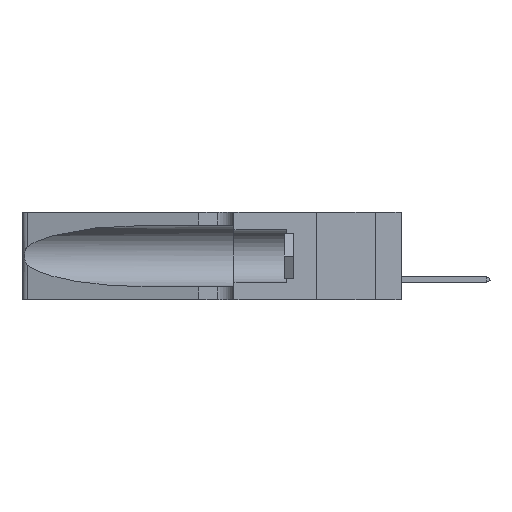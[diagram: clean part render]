
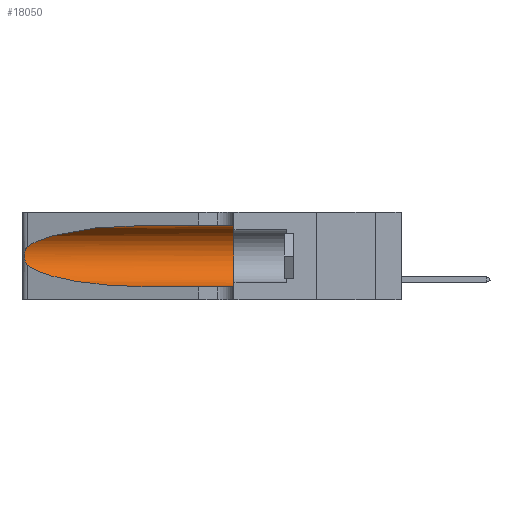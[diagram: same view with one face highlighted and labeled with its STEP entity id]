
A CAD part, left-side view. The second image highlights one B-rep face of the part: STEP entity #18050.
In plain terms, the highlighted cylindrical face has radius 3.308 mm (diameter 6.617 mm), a partial arc.
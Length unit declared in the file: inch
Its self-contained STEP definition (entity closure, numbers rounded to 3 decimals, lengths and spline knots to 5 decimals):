
#1642 = CIRCLE ( 'NONE', #11534, 0.13025 ) ;
#1746 = CARTESIAN_POINT ( 'NONE',  ( 0.26075, 1.23896, 0.19203 ) ) ;
#3138 = VERTEX_POINT ( 'NONE', #9955 ) ;
#3165 = EDGE_CURVE ( 'NONE', #3138, #22625, #1642, .T. ) ;
#3454 = VERTEX_POINT ( 'NONE', #5113 ) ;
#3626 = CARTESIAN_POINT ( 'NONE',  ( 0.25789, 1.23486, 0.15765 ) ) ;
#4269 = ORIENTED_EDGE ( 'NONE', *, *, #8485, .T. ) ;
#5087 = CARTESIAN_POINT ( 'NONE',  ( 0.25487, 1.22718, 0.22369 ) ) ;
#5113 = CARTESIAN_POINT ( 'NONE',  ( 0.25487, 1.22718, 0.22369 ) ) ;
#5138 = VERTEX_POINT ( 'NONE', #9258 ) ;
#5312 = CARTESIAN_POINT ( 'NONE',  ( 0.26018, 1.23835, 0.19895 ) ) ;
#5624 = CARTESIAN_POINT ( 'NONE',  ( 0.1305, 1.61858, 0.05475 ) ) ;
#5679 = ORIENTED_EDGE ( 'NONE', *, *, #8250, .F. ) ;
#5710 = DIRECTION ( 'NONE',  ( 0., -1., 0. ) ) ;
#6046 = LINE ( 'NONE', #5624, #17966 ) ;
#6229 = CARTESIAN_POINT ( 'NONE',  ( 0.1305, 0.35, 0.185 ) ) ;
#7249 = CARTESIAN_POINT ( 'NONE',  ( 0.26075, 1.23896, 0.178 ) ) ;
#7767 = EDGE_LOOP ( 'NONE', ( #4269, #24667, #21791, #23606, #15381, #5679 ) ) ;
#8250 = EDGE_CURVE ( 'NONE', #21780, #3138, #8544, .T. ) ;
#8485 = EDGE_CURVE ( 'NONE', #21780, #3454, #23992, .T. ) ;
#8544 = LINE ( 'NONE', #18315, #16894 ) ;
#9237 = CARTESIAN_POINT ( 'NONE',  ( 0.26017, 1.23833, 0.17102 ) ) ;
#9258 = CARTESIAN_POINT ( 'NONE',  ( 0.25487, 1.22718, 0.14631 ) ) ;
#9955 = CARTESIAN_POINT ( 'NONE',  ( 0.1305, 0.35, 0.31525 ) ) ;
#10223 = DIRECTION ( 'NONE',  ( 0., 0., -1. ) ) ;
#10801 = VERTEX_POINT ( 'NONE', #18827 ) ;
#11534 = AXIS2_PLACEMENT_3D ( 'NONE', #6229, #17575, #21501 ) ;
#11872 = CARTESIAN_POINT ( 'NONE',  ( 0.2373, 1.15595, 0.08982 ) ) ;
#12043 = CARTESIAN_POINT ( 'NONE',  ( 0.25487, 1.22718, 0.14631 ) ) ;
#12733 = CARTESIAN_POINT ( 'NONE',  ( 0.2373, 1.15595, 0.28018 ) ) ;
#13086 = CARTESIAN_POINT ( 'NONE',  ( 0.25639, 1.23186, 0.15144 ) ) ;
#13724 = CARTESIAN_POINT ( 'NONE',  ( 0.18966, 0.96281, 0.05475 ) ) ;
#14057 = CARTESIAN_POINT ( 'NONE',  ( 0.1305, 0.72297, 0.05475 ) ) ;
#14345 = AXIS2_PLACEMENT_3D ( 'NONE', #23472, #23643, #10223 ) ;
#14842 = CARTESIAN_POINT ( 'NONE',  ( 0.1305, 0.72297, 0.31525 ) ) ;
#14890 = CARTESIAN_POINT ( 'NONE',  ( 0.18966, 0.96281, 0.31525 ) ) ;
#14919 = CARTESIAN_POINT ( 'NONE',  ( 0.25787, 1.23484, 0.2124 ) ) ;
#15381 = ORIENTED_EDGE ( 'NONE', *, *, #3165, .F. ) ;
#16384 = B_SPLINE_CURVE_WITH_KNOTS ( 'NONE', 3,
 ( #20763, #20840, #20672, #14919, #20518, #5312, #1746, #7249, #9237, #22579, #3626, #13086, #20601, #22663 ),
 .UNSPECIFIED., .F., .F.,
 ( 4, 2, 2, 2, 2, 2, 4 ),
 ( 0., 0.00027, 0.00053, 0.00107, 0.0016, 0.00187, 0.00214 ),
 .UNSPECIFIED. ) ;
#16664 = EDGE_CURVE ( 'NONE', #5138, #10801, #22330, .T. ) ;
#16770 = CARTESIAN_POINT ( 'NONE',  ( 0.1305, 0.35, 0.05475 ) ) ;
#16894 = VECTOR ( 'NONE', #24023, 39.37008 ) ;
#17575 = DIRECTION ( 'NONE',  ( 0., 1., 0. ) ) ;
#17966 = VECTOR ( 'NONE', #5710, 39.37008 ) ;
#18050 = ADVANCED_FACE ( 'NONE', ( #18690 ), #21098, .F. ) ;
#18315 = CARTESIAN_POINT ( 'NONE',  ( 0.1305, 1.61858, 0.31525 ) ) ;
#18690 = FACE_OUTER_BOUND ( 'NONE', #7767, .T. ) ;
#18827 = CARTESIAN_POINT ( 'NONE',  ( 0.1305, 0.72297, 0.05475 ) ) ;
#20518 = CARTESIAN_POINT ( 'NONE',  ( 0.25854, 1.2359, 0.20912 ) ) ;
#20556 = EDGE_CURVE ( 'NONE', #10801, #22625, #6046, .T. ) ;
#20601 = CARTESIAN_POINT ( 'NONE',  ( 0.25555, 1.22993, 0.14849 ) ) ;
#20672 = CARTESIAN_POINT ( 'NONE',  ( 0.25639, 1.23184, 0.21858 ) ) ;
#20763 = CARTESIAN_POINT ( 'NONE',  ( 0.25487, 1.22718, 0.22369 ) ) ;
#20840 = CARTESIAN_POINT ( 'NONE',  ( 0.25555, 1.22994, 0.2215 ) ) ;
#21098 = CYLINDRICAL_SURFACE ( 'NONE', #14345, 0.13025 ) ;
#21501 = DIRECTION ( 'NONE',  ( 0., 0., 1. ) ) ;
#21758 = EDGE_CURVE ( 'NONE', #3454, #5138, #16384, .T. ) ;
#21780 = VERTEX_POINT ( 'NONE', #14842 ) ;
#21791 = ORIENTED_EDGE ( 'NONE', *, *, #16664, .T. ) ;
#22330 =( BOUNDED_CURVE ( )  B_SPLINE_CURVE ( 3, ( #12043, #11872, #13724, #14057 ),
 .UNSPECIFIED., .F., .F. ) 
 B_SPLINE_CURVE_WITH_KNOTS ( ( 4, 4 ),
 ( 3.44316, 4.71239 ),
 .UNSPECIFIED. ) 
 CURVE ( )  GEOMETRIC_REPRESENTATION_ITEM ( )  RATIONAL_B_SPLINE_CURVE ( ( 1., 0.87, 0.87, 1. ) ) 
 REPRESENTATION_ITEM ( '' )  );
#22579 = CARTESIAN_POINT ( 'NONE',  ( 0.25856, 1.23593, 0.16098 ) ) ;
#22625 = VERTEX_POINT ( 'NONE', #16770 ) ;
#22663 = CARTESIAN_POINT ( 'NONE',  ( 0.25487, 1.22718, 0.14631 ) ) ;
#23472 = CARTESIAN_POINT ( 'NONE',  ( 0.1305, 1.61858, 0.185 ) ) ;
#23606 = ORIENTED_EDGE ( 'NONE', *, *, #20556, .T. ) ;
#23643 = DIRECTION ( 'NONE',  ( 0., -1., 0. ) ) ;
#23992 =( BOUNDED_CURVE ( )  B_SPLINE_CURVE ( 3, ( #24101, #14890, #12733, #5087 ),
 .UNSPECIFIED., .F., .F. ) 
 B_SPLINE_CURVE_WITH_KNOTS ( ( 4, 4 ),
 ( 1.5708, 2.84003 ),
 .UNSPECIFIED. ) 
 CURVE ( )  GEOMETRIC_REPRESENTATION_ITEM ( )  RATIONAL_B_SPLINE_CURVE ( ( 1., 0.87, 0.87, 1. ) ) 
 REPRESENTATION_ITEM ( '' )  );
#24023 = DIRECTION ( 'NONE',  ( 0., -1., 0. ) ) ;
#24101 = CARTESIAN_POINT ( 'NONE',  ( 0.1305, 0.72297, 0.31525 ) ) ;
#24667 = ORIENTED_EDGE ( 'NONE', *, *, #21758, .T. ) ;
